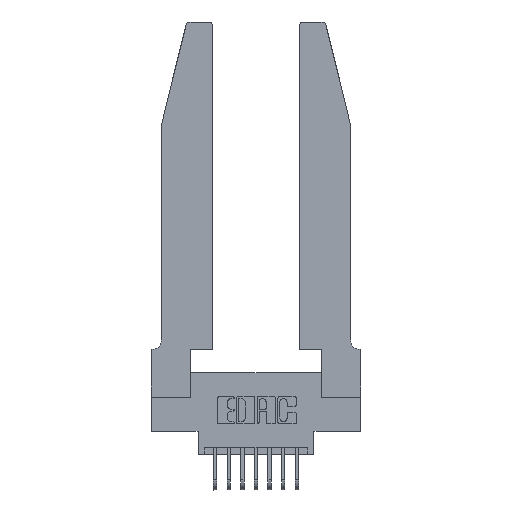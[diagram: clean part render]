
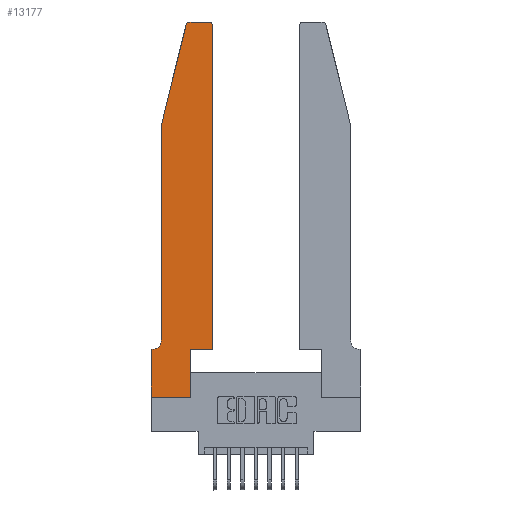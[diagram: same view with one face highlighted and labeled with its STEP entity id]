
A CAD part, top view. The second image highlights one B-rep face of the part: STEP entity #13177.
In plain terms, the highlighted planar face has unit normal (0, 0, 1).
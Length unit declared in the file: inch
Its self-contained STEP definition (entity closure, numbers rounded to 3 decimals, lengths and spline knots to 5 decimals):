
#304 = LINE ( 'NONE', #6857, #8877 ) ;
#314 = VERTEX_POINT ( 'NONE', #9492 ) ;
#462 = EDGE_CURVE ( 'NONE', #9963, #3087, #2873, .T. ) ;
#490 = DIRECTION ( 'NONE',  ( 0., 0., 1. ) ) ;
#806 = VERTEX_POINT ( 'NONE', #4792 ) ;
#985 = CARTESIAN_POINT ( 'NONE',  ( 0.0055, 0.35, 0.37 ) ) ;
#1052 = CARTESIAN_POINT ( 'NONE',  ( 0.4505, 2.72, 0.37 ) ) ;
#1626 = EDGE_CURVE ( 'NONE', #9001, #6499, #3020, .T. ) ;
#1646 = EDGE_CURVE ( 'NONE', #8518, #6400, #304, .T. ) ;
#1881 = ORIENTED_EDGE ( 'NONE', *, *, #5042, .T. ) ;
#1929 = ORIENTED_EDGE ( 'NONE', *, *, #13842, .T. ) ;
#1954 = CARTESIAN_POINT ( 'NONE',  ( 0., 0., 0.37 ) ) ;
#1956 = VECTOR ( 'NONE', #13695, 39.37008 ) ;
#2212 = CARTESIAN_POINT ( 'NONE',  ( 0.0755, 2., 0.37 ) ) ;
#2421 = DIRECTION ( 'NONE',  ( 0., 0., 1. ) ) ;
#2734 = LINE ( 'NONE', #3523, #8605 ) ;
#2873 = LINE ( 'NONE', #4191, #14793 ) ;
#2910 = DIRECTION ( 'NONE',  ( 0., 0., -1. ) ) ;
#2965 = EDGE_CURVE ( 'NONE', #11818, #9963, #14721, .T. ) ;
#3020 = LINE ( 'NONE', #10169, #14931 ) ;
#3036 = CARTESIAN_POINT ( 'NONE',  ( 0.0055, 0.42, 0.37 ) ) ;
#3087 = VERTEX_POINT ( 'NONE', #14217 ) ;
#3127 = DIRECTION ( 'NONE',  ( 0., -1., 0. ) ) ;
#3478 = CARTESIAN_POINT ( 'NONE',  ( 0.284, 2.75, 0.37 ) ) ;
#3523 = CARTESIAN_POINT ( 'NONE',  ( 0.2605, 2.75, 0.37 ) ) ;
#3699 = DIRECTION ( 'NONE',  ( -1., 0., 0. ) ) ;
#4191 = CARTESIAN_POINT ( 'NONE',  ( 0.0755, 0.35, 0.37 ) ) ;
#4488 = DIRECTION ( 'NONE',  ( -1., 0., 0. ) ) ;
#4522 = VERTEX_POINT ( 'NONE', #7760 ) ;
#4533 = ORIENTED_EDGE ( 'NONE', *, *, #12038, .T. ) ;
#4792 = CARTESIAN_POINT ( 'NONE',  ( 0.25487, 2.72718, 0.37 ) ) ;
#4970 = ORIENTED_EDGE ( 'NONE', *, *, #10097, .T. ) ;
#5042 = EDGE_CURVE ( 'NONE', #6042, #806, #6352, .T. ) ;
#5086 = LINE ( 'NONE', #12566, #1956 ) ;
#5560 = CARTESIAN_POINT ( 'NONE',  ( 0., 0.35, 0.37 ) ) ;
#5571 = ORIENTED_EDGE ( 'NONE', *, *, #1626, .T. ) ;
#5811 = CARTESIAN_POINT ( 'NONE',  ( 0.0755, 2., 0.37 ) ) ;
#5849 = CIRCLE ( 'NONE', #8652, 0.03 ) ;
#6042 = VERTEX_POINT ( 'NONE', #3478 ) ;
#6203 = LINE ( 'NONE', #5811, #11347 ) ;
#6352 = CIRCLE ( 'NONE', #10138, 0.03 ) ;
#6400 = VERTEX_POINT ( 'NONE', #1052 ) ;
#6420 = ORIENTED_EDGE ( 'NONE', *, *, #1646, .T. ) ;
#6499 = VERTEX_POINT ( 'NONE', #12891 ) ;
#6631 = DIRECTION ( 'NONE',  ( 1., 0., 0. ) ) ;
#6734 = DIRECTION ( 'NONE',  ( 0., 0., 1. ) ) ;
#6742 = ORIENTED_EDGE ( 'NONE', *, *, #2965, .T. ) ;
#6839 = ORIENTED_EDGE ( 'NONE', *, *, #11837, .T. ) ;
#6857 = CARTESIAN_POINT ( 'NONE',  ( 0.4505, 0.35, 0.37 ) ) ;
#6894 = DIRECTION ( 'NONE',  ( 0., 1., 0. ) ) ;
#6981 = LINE ( 'NONE', #12062, #9702 ) ;
#6995 = DIRECTION ( 'NONE',  ( 0., -1., 0. ) ) ;
#7478 = DIRECTION ( 'NONE',  ( -0.239, -0.971, 0. ) ) ;
#7509 = CARTESIAN_POINT ( 'NONE',  ( 0.284, 2.72, 0.37 ) ) ;
#7543 = LINE ( 'NONE', #1954, #13655 ) ;
#7760 = CARTESIAN_POINT ( 'NONE',  ( 0.4205, 2.75, 0.37 ) ) ;
#8518 = VERTEX_POINT ( 'NONE', #11195 ) ;
#8581 = CARTESIAN_POINT ( 'NONE',  ( 0.0755, 0.42, 0.37 ) ) ;
#8605 = VECTOR ( 'NONE', #10526, 39.37008 ) ;
#8652 = AXIS2_PLACEMENT_3D ( 'NONE', #9411, #2421, #10573 ) ;
#8662 = DIRECTION ( 'NONE',  ( 1., 0., 0. ) ) ;
#8857 = AXIS2_PLACEMENT_3D ( 'NONE', #5560, #6734, #14751 ) ;
#8877 = VECTOR ( 'NONE', #6894, 39.37008 ) ;
#9001 = VERTEX_POINT ( 'NONE', #9244 ) ;
#9244 = CARTESIAN_POINT ( 'NONE',  ( 0., 0., 0.37 ) ) ;
#9350 = EDGE_LOOP ( 'NONE', ( #10376, #1881, #6839, #10094, #6742, #9819, #4533, #5571, #11917, #1929, #6420, #4970 ) ) ;
#9411 = CARTESIAN_POINT ( 'NONE',  ( 0.4205, 2.72, 0.37 ) ) ;
#9492 = CARTESIAN_POINT ( 'NONE',  ( 0.2865, 0.35, 0.37 ) ) ;
#9702 = VECTOR ( 'NONE', #7478, 39.37008 ) ;
#9819 = ORIENTED_EDGE ( 'NONE', *, *, #462, .T. ) ;
#9963 = VERTEX_POINT ( 'NONE', #985 ) ;
#10094 = ORIENTED_EDGE ( 'NONE', *, *, #13312, .T. ) ;
#10096 = EDGE_CURVE ( 'NONE', #4522, #6042, #2734, .T. ) ;
#10097 = EDGE_CURVE ( 'NONE', #6400, #4522, #5849, .T. ) ;
#10138 = AXIS2_PLACEMENT_3D ( 'NONE', #7509, #490, #8662 ) ;
#10169 = CARTESIAN_POINT ( 'NONE',  ( 0., 0., 0.37 ) ) ;
#10324 = DIRECTION ( 'NONE',  ( 0., 1., 0. ) ) ;
#10376 = ORIENTED_EDGE ( 'NONE', *, *, #10096, .T. ) ;
#10526 = DIRECTION ( 'NONE',  ( -1., 0., 0. ) ) ;
#10573 = DIRECTION ( 'NONE',  ( 1., 0., 0. ) ) ;
#11112 = FACE_OUTER_BOUND ( 'NONE', #9350, .T. ) ;
#11136 = VECTOR ( 'NONE', #10324, 39.37008 ) ;
#11195 = CARTESIAN_POINT ( 'NONE',  ( 0.4505, 0.35, 0.37 ) ) ;
#11347 = VECTOR ( 'NONE', #6995, 39.37008 ) ;
#11818 = VERTEX_POINT ( 'NONE', #8581 ) ;
#11837 = EDGE_CURVE ( 'NONE', #806, #12172, #6981, .T. ) ;
#11917 = ORIENTED_EDGE ( 'NONE', *, *, #12145, .T. ) ;
#12038 = EDGE_CURVE ( 'NONE', #3087, #9001, #7543, .T. ) ;
#12062 = CARTESIAN_POINT ( 'NONE',  ( 0.0755, 2., 0.37 ) ) ;
#12145 = EDGE_CURVE ( 'NONE', #6499, #314, #14174, .T. ) ;
#12172 = VERTEX_POINT ( 'NONE', #2212 ) ;
#12566 = CARTESIAN_POINT ( 'NONE',  ( 0.4505, 0.35, 0.37 ) ) ;
#12615 = CARTESIAN_POINT ( 'NONE',  ( 0.2865, 0.35, 0.37 ) ) ;
#12891 = CARTESIAN_POINT ( 'NONE',  ( 0.2865, 0., 0.37 ) ) ;
#13177 = ADVANCED_FACE ( 'NONE', ( #11112 ), #13660, .T. ) ;
#13312 = EDGE_CURVE ( 'NONE', #12172, #11818, #6203, .T. ) ;
#13655 = VECTOR ( 'NONE', #3127, 39.37008 ) ;
#13660 = PLANE ( 'NONE',  #8857 ) ;
#13695 = DIRECTION ( 'NONE',  ( 1., 0., 0. ) ) ;
#13842 = EDGE_CURVE ( 'NONE', #314, #8518, #5086, .T. ) ;
#14174 = LINE ( 'NONE', #12615, #11136 ) ;
#14217 = CARTESIAN_POINT ( 'NONE',  ( 0., 0.35, 0.37 ) ) ;
#14371 = AXIS2_PLACEMENT_3D ( 'NONE', #3036, #2910, #3699 ) ;
#14721 = CIRCLE ( 'NONE', #14371, 0.07 ) ;
#14751 = DIRECTION ( 'NONE',  ( 1., 0., 0. ) ) ;
#14793 = VECTOR ( 'NONE', #4488, 39.37008 ) ;
#14931 = VECTOR ( 'NONE', #6631, 39.37008 ) ;
